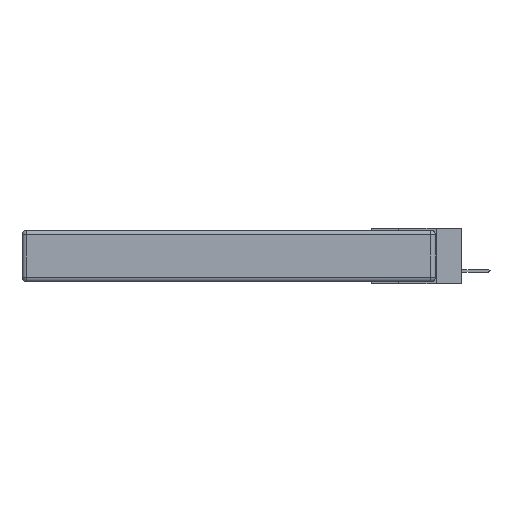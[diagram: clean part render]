
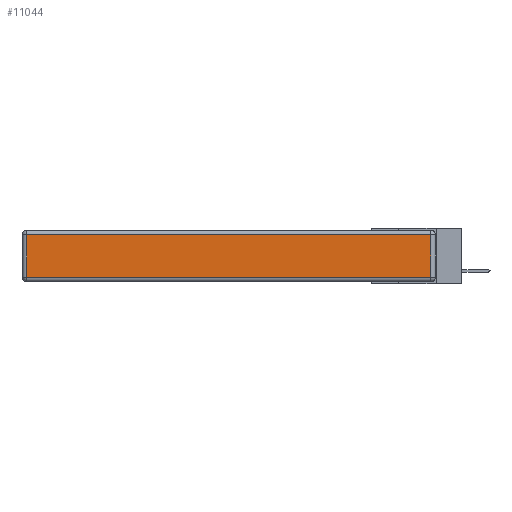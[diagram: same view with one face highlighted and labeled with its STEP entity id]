
A CAD part, left-side view. The second image highlights one B-rep face of the part: STEP entity #11044.
In plain terms, the highlighted planar face has unit normal (-1, 0, 0).
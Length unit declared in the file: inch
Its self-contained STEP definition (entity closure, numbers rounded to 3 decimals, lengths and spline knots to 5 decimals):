
#370 = EDGE_CURVE ( 'NONE', #1654, #11516, #15057, .T. ) ;
#621 = ORIENTED_EDGE ( 'NONE', *, *, #1039, .T. ) ;
#1039 = EDGE_CURVE ( 'NONE', #20209, #1654, #4877, .T. ) ;
#1234 = FACE_OUTER_BOUND ( 'NONE', #6481, .T. ) ;
#1392 = DIRECTION ( 'NONE',  ( 0., -1., 0. ) ) ;
#1431 = CARTESIAN_POINT ( 'NONE',  ( 0., 0.03, -0.03 ) ) ;
#1621 = VERTEX_POINT ( 'NONE', #1431 ) ;
#1654 = VERTEX_POINT ( 'NONE', #19579 ) ;
#3658 = PLANE ( 'NONE',  #19188 ) ;
#4877 = LINE ( 'NONE', #15377, #15314 ) ;
#5444 = DIRECTION ( 'NONE',  ( 0., 1., 0. ) ) ;
#5619 = CARTESIAN_POINT ( 'NONE',  ( 0., 2.75, -0.03 ) ) ;
#5646 = CARTESIAN_POINT ( 'NONE',  ( 0., 0.03, -0.343 ) ) ;
#6481 = EDGE_LOOP ( 'NONE', ( #16349, #24097, #13076, #621 ) ) ;
#7200 = VECTOR ( 'NONE', #5444, 39.37008 ) ;
#7462 = VECTOR ( 'NONE', #1392, 39.37008 ) ;
#7605 = EDGE_CURVE ( 'NONE', #1621, #20209, #13537, .T. ) ;
#7789 = DIRECTION ( 'NONE',  ( 0., 0., 1. ) ) ;
#10193 = CARTESIAN_POINT ( 'NONE',  ( 0., 0., -0.343 ) ) ;
#10927 = VECTOR ( 'NONE', #21897, 39.37008 ) ;
#11044 = ADVANCED_FACE ( 'NONE', ( #1234 ), #3658, .T. ) ;
#11516 = VERTEX_POINT ( 'NONE', #12136 ) ;
#12136 = CARTESIAN_POINT ( 'NONE',  ( 0., 0.03, -0.313 ) ) ;
#13076 = ORIENTED_EDGE ( 'NONE', *, *, #7605, .T. ) ;
#13537 = LINE ( 'NONE', #5619, #7200 ) ;
#13702 = EDGE_CURVE ( 'NONE', #11516, #1621, #24178, .T. ) ;
#15057 = LINE ( 'NONE', #24628, #7462 ) ;
#15314 = VECTOR ( 'NONE', #21546, 39.37008 ) ;
#15377 = CARTESIAN_POINT ( 'NONE',  ( 0., 2.72, -0.343 ) ) ;
#16349 = ORIENTED_EDGE ( 'NONE', *, *, #370, .T. ) ;
#18055 = CARTESIAN_POINT ( 'NONE',  ( 0., 2.72, -0.03 ) ) ;
#18210 = DIRECTION ( 'NONE',  ( -1., 0., 0. ) ) ;
#19188 = AXIS2_PLACEMENT_3D ( 'NONE', #10193, #18210, #7789 ) ;
#19579 = CARTESIAN_POINT ( 'NONE',  ( 0., 2.72, -0.313 ) ) ;
#20209 = VERTEX_POINT ( 'NONE', #18055 ) ;
#21546 = DIRECTION ( 'NONE',  ( 0., 0., -1. ) ) ;
#21897 = DIRECTION ( 'NONE',  ( 0., 0., 1. ) ) ;
#24097 = ORIENTED_EDGE ( 'NONE', *, *, #13702, .T. ) ;
#24178 = LINE ( 'NONE', #5646, #10927 ) ;
#24628 = CARTESIAN_POINT ( 'NONE',  ( 0., 0., -0.313 ) ) ;
